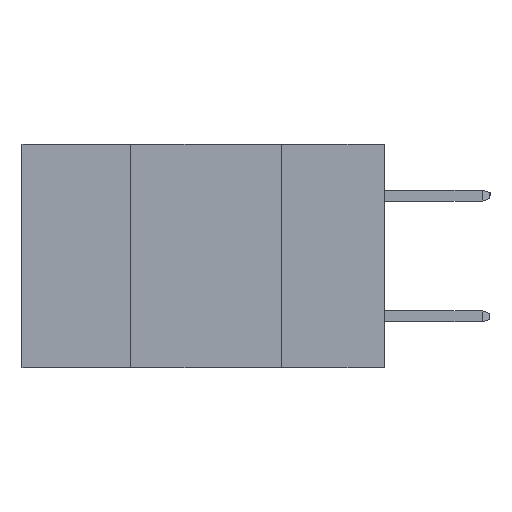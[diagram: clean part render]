
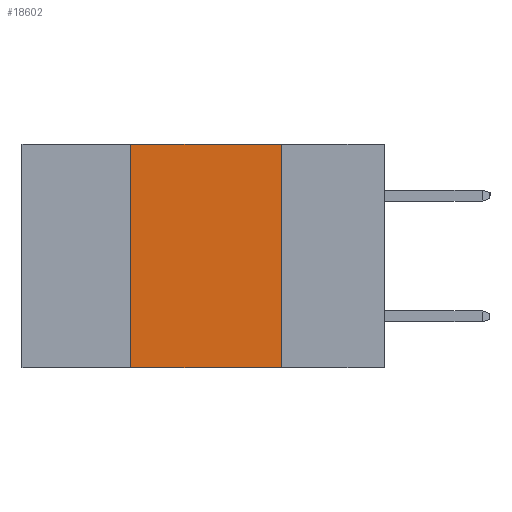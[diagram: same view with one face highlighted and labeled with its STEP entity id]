
A CAD part, left-side view. The second image highlights one B-rep face of the part: STEP entity #18602.
In plain terms, the highlighted planar face has unit normal (-1, 0, 0).
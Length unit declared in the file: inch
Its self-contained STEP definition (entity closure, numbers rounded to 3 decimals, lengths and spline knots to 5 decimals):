
#417 = VECTOR ( 'NONE', #1619, 39.37008 ) ;
#1034 = CARTESIAN_POINT ( 'NONE',  ( 0., 0.42, -0.37 ) ) ;
#1619 = DIRECTION ( 'NONE',  ( 0., -1., 0. ) ) ;
#2633 = ORIENTED_EDGE ( 'NONE', *, *, #22515, .T. ) ;
#3745 = LINE ( 'NONE', #12619, #9521 ) ;
#4254 = EDGE_CURVE ( 'NONE', #8714, #8439, #5691, .T. ) ;
#4558 = VERTEX_POINT ( 'NONE', #11488 ) ;
#4824 = CARTESIAN_POINT ( 'NONE',  ( 0., 0.42, 0. ) ) ;
#5691 = LINE ( 'NONE', #16199, #17765 ) ;
#5947 = CARTESIAN_POINT ( 'NONE',  ( 0., 0.6, -0.37 ) ) ;
#7895 = LINE ( 'NONE', #5947, #417 ) ;
#8439 = VERTEX_POINT ( 'NONE', #24106 ) ;
#8714 = VERTEX_POINT ( 'NONE', #4824 ) ;
#9521 = VECTOR ( 'NONE', #10261, 39.37008 ) ;
#10261 = DIRECTION ( 'NONE',  ( 0., 0., -1. ) ) ;
#10782 = PLANE ( 'NONE',  #19356 ) ;
#11488 = CARTESIAN_POINT ( 'NONE',  ( 0., 0.17, -0.37 ) ) ;
#12236 = EDGE_CURVE ( 'NONE', #8439, #4558, #3745, .T. ) ;
#12619 = CARTESIAN_POINT ( 'NONE',  ( 0., 0.17, -0.37 ) ) ;
#12921 = EDGE_LOOP ( 'NONE', ( #21163, #21254, #21509, #2633 ) ) ;
#14107 = VECTOR ( 'NONE', #15013, 39.37008 ) ;
#15013 = DIRECTION ( 'NONE',  ( 0., 0., 1. ) ) ;
#16199 = CARTESIAN_POINT ( 'NONE',  ( 0., 0.6, 0. ) ) ;
#17088 = LINE ( 'NONE', #25549, #14107 ) ;
#17552 = CARTESIAN_POINT ( 'NONE',  ( 0., 0.6, 0. ) ) ;
#17765 = VECTOR ( 'NONE', #26484, 39.37008 ) ;
#18602 = ADVANCED_FACE ( 'NONE', ( #23657 ), #10782, .F. ) ;
#19211 = DIRECTION ( 'NONE',  ( 0., 0., -1. ) ) ;
#19344 = DIRECTION ( 'NONE',  ( 1., 0., 0. ) ) ;
#19356 = AXIS2_PLACEMENT_3D ( 'NONE', #17552, #19344, #19211 ) ;
#19926 = EDGE_CURVE ( 'NONE', #22958, #8714, #17088, .T. ) ;
#21163 = ORIENTED_EDGE ( 'NONE', *, *, #12236, .F. ) ;
#21254 = ORIENTED_EDGE ( 'NONE', *, *, #4254, .F. ) ;
#21509 = ORIENTED_EDGE ( 'NONE', *, *, #19926, .F. ) ;
#22515 = EDGE_CURVE ( 'NONE', #22958, #4558, #7895, .T. ) ;
#22958 = VERTEX_POINT ( 'NONE', #1034 ) ;
#23657 = FACE_OUTER_BOUND ( 'NONE', #12921, .T. ) ;
#24106 = CARTESIAN_POINT ( 'NONE',  ( 0., 0.17, 0. ) ) ;
#25549 = CARTESIAN_POINT ( 'NONE',  ( 0., 0.42, -0.37 ) ) ;
#26484 = DIRECTION ( 'NONE',  ( 0., -1., 0. ) ) ;
